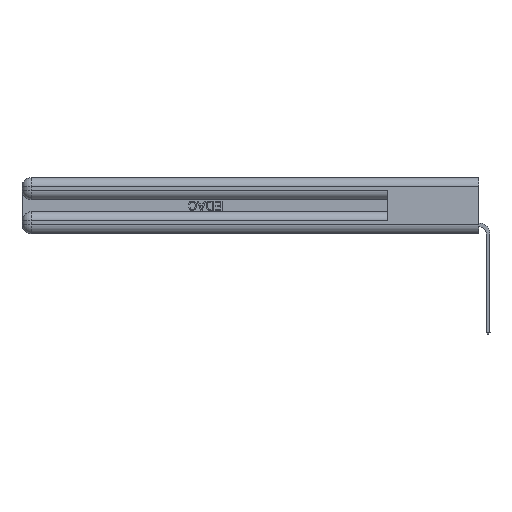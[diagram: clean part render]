
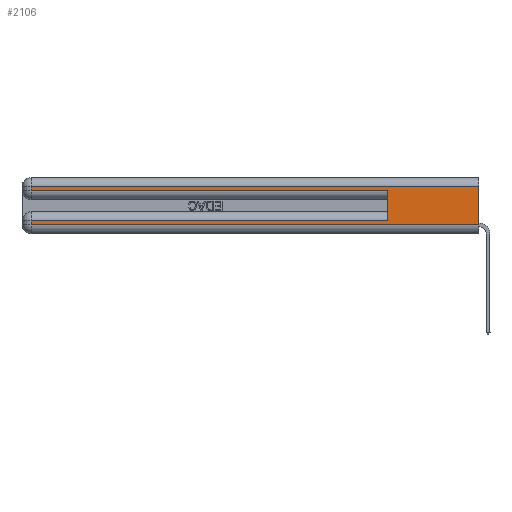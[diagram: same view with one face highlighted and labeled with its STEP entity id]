
A CAD part, left-side view. The second image highlights one B-rep face of the part: STEP entity #2106.
In plain terms, the highlighted planar face has unit normal (-1, 0, 0).
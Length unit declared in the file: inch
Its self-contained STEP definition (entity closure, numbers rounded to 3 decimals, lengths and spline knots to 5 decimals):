
#337 = VECTOR ( 'NONE', #29522, 39.37008 ) ;
#367 = ORIENTED_EDGE ( 'NONE', *, *, #8118, .T. ) ;
#1357 = ORIENTED_EDGE ( 'NONE', *, *, #17397, .F. ) ;
#2106 = ADVANCED_FACE ( 'NONE', ( #3311 ), #14088, .F. ) ;
#2577 = CARTESIAN_POINT ( 'NONE',  ( 0., 0.6, 0.145 ) ) ;
#3243 = LINE ( 'NONE', #16745, #8415 ) ;
#3311 = FACE_OUTER_BOUND ( 'NONE', #9357, .T. ) ;
#3483 = CARTESIAN_POINT ( 'NONE',  ( 0., 2.94, 0.31 ) ) ;
#3484 = CARTESIAN_POINT ( 'NONE',  ( 0., 0., 0.31 ) ) ;
#3765 = CARTESIAN_POINT ( 'NONE',  ( 0., 0., 0.285 ) ) ;
#4821 = DIRECTION ( 'NONE',  ( 0., 0., -1. ) ) ;
#5753 = DIRECTION ( 'NONE',  ( 0., 1., 0. ) ) ;
#6178 = EDGE_CURVE ( 'NONE', #17899, #22546, #12957, .T. ) ;
#7715 = EDGE_CURVE ( 'NONE', #25433, #18146, #8040, .T. ) ;
#7836 = VERTEX_POINT ( 'NONE', #17473 ) ;
#8005 = VECTOR ( 'NONE', #5753, 39.37008 ) ;
#8040 = LINE ( 'NONE', #3484, #21487 ) ;
#8118 = EDGE_CURVE ( 'NONE', #17899, #7836, #8817, .T. ) ;
#8415 = VECTOR ( 'NONE', #29456, 39.37008 ) ;
#8817 = LINE ( 'NONE', #10960, #8005 ) ;
#9357 = EDGE_LOOP ( 'NONE', ( #1357, #29558, #32507, #27709, #31980, #367, #27962, #14387 ) ) ;
#10366 = VERTEX_POINT ( 'NONE', #12812 ) ;
#10960 = CARTESIAN_POINT ( 'NONE',  ( 0., 0., 0.085 ) ) ;
#11288 = CARTESIAN_POINT ( 'NONE',  ( 0., 0., 0.31 ) ) ;
#11682 = DIRECTION ( 'NONE',  ( 0., 0., -1. ) ) ;
#12479 = CARTESIAN_POINT ( 'NONE',  ( 0., 2.94, 0.37 ) ) ;
#12592 = CARTESIAN_POINT ( 'NONE',  ( 0., 0., 0.06 ) ) ;
#12812 = CARTESIAN_POINT ( 'NONE',  ( 0., 0., 0.06 ) ) ;
#12957 = LINE ( 'NONE', #2577, #18071 ) ;
#13576 = DIRECTION ( 'NONE',  ( 0., 1., 0. ) ) ;
#13854 = LINE ( 'NONE', #3765, #337 ) ;
#14088 = PLANE ( 'NONE',  #30489 ) ;
#14320 = LINE ( 'NONE', #12592, #31326 ) ;
#14387 = ORIENTED_EDGE ( 'NONE', *, *, #19066, .T. ) ;
#15103 = DIRECTION ( 'NONE',  ( 0., -1., 0. ) ) ;
#15558 = VERTEX_POINT ( 'NONE', #25946 ) ;
#15999 = CARTESIAN_POINT ( 'NONE',  ( 0., 0.6, 0.285 ) ) ;
#16745 = CARTESIAN_POINT ( 'NONE',  ( 0., 2.94, 0.37 ) ) ;
#17206 = VECTOR ( 'NONE', #4821, 39.37008 ) ;
#17397 = EDGE_CURVE ( 'NONE', #25433, #10366, #21546, .T. ) ;
#17473 = CARTESIAN_POINT ( 'NONE',  ( 0., 2.94, 0.085 ) ) ;
#17899 = VERTEX_POINT ( 'NONE', #30368 ) ;
#18071 = VECTOR ( 'NONE', #25330, 39.37008 ) ;
#18146 = VERTEX_POINT ( 'NONE', #3483 ) ;
#19066 = EDGE_CURVE ( 'NONE', #15558, #10366, #14320, .T. ) ;
#20140 = EDGE_CURVE ( 'NONE', #21981, #22546, #13854, .T. ) ;
#20754 = VECTOR ( 'NONE', #27618, 39.37008 ) ;
#21487 = VECTOR ( 'NONE', #13576, 39.37008 ) ;
#21546 = LINE ( 'NONE', #22556, #20754 ) ;
#21981 = VERTEX_POINT ( 'NONE', #31169 ) ;
#22546 = VERTEX_POINT ( 'NONE', #15999 ) ;
#22556 = CARTESIAN_POINT ( 'NONE',  ( 0., 0., 0.37 ) ) ;
#22832 = EDGE_CURVE ( 'NONE', #18146, #21981, #24701, .T. ) ;
#24701 = LINE ( 'NONE', #12479, #17206 ) ;
#25330 = DIRECTION ( 'NONE',  ( 0., 0., 1. ) ) ;
#25433 = VERTEX_POINT ( 'NONE', #11288 ) ;
#25946 = CARTESIAN_POINT ( 'NONE',  ( 0., 2.94, 0.06 ) ) ;
#26777 = DIRECTION ( 'NONE',  ( 1., 0., 0. ) ) ;
#27618 = DIRECTION ( 'NONE',  ( 0., 0., -1. ) ) ;
#27709 = ORIENTED_EDGE ( 'NONE', *, *, #20140, .T. ) ;
#27962 = ORIENTED_EDGE ( 'NONE', *, *, #29617, .T. ) ;
#29456 = DIRECTION ( 'NONE',  ( 0., 0., -1. ) ) ;
#29522 = DIRECTION ( 'NONE',  ( 0., -1., 0. ) ) ;
#29558 = ORIENTED_EDGE ( 'NONE', *, *, #7715, .T. ) ;
#29617 = EDGE_CURVE ( 'NONE', #7836, #15558, #3243, .T. ) ;
#30368 = CARTESIAN_POINT ( 'NONE',  ( 0., 0.6, 0.085 ) ) ;
#30489 = AXIS2_PLACEMENT_3D ( 'NONE', #31755, #26777, #11682 ) ;
#31169 = CARTESIAN_POINT ( 'NONE',  ( 0., 2.94, 0.285 ) ) ;
#31326 = VECTOR ( 'NONE', #15103, 39.37008 ) ;
#31755 = CARTESIAN_POINT ( 'NONE',  ( 0., 0., 0.37 ) ) ;
#31980 = ORIENTED_EDGE ( 'NONE', *, *, #6178, .F. ) ;
#32507 = ORIENTED_EDGE ( 'NONE', *, *, #22832, .T. ) ;
